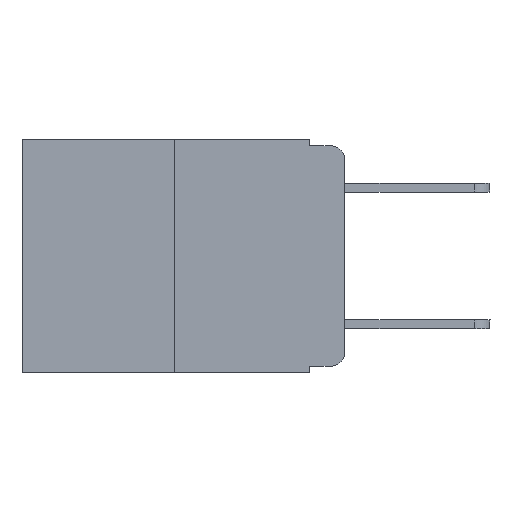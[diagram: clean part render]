
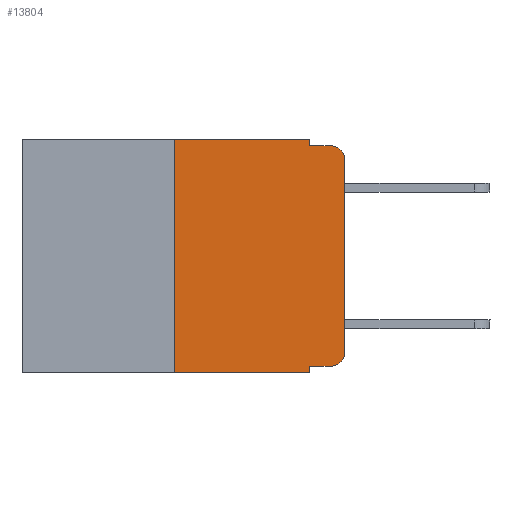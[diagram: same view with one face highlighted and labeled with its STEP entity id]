
A CAD part, left-side view. The second image highlights one B-rep face of the part: STEP entity #13804.
In plain terms, the highlighted planar face has unit normal (-1, 0, 0).
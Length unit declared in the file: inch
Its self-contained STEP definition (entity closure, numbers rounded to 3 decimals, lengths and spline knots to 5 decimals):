
#73 = LINE ( 'NONE', #9291, #13751 ) ;
#338 = CARTESIAN_POINT ( 'NONE',  ( 0., 0.051, -0.333 ) ) ;
#714 = CARTESIAN_POINT ( 'NONE',  ( 0., 0.051, -0.01 ) ) ;
#1310 = VECTOR ( 'NONE', #9167, 39.37008 ) ;
#1351 = DIRECTION ( 'NONE',  ( 0., 0., 1. ) ) ;
#1710 = DIRECTION ( 'NONE',  ( 0., 0., -1. ) ) ;
#1842 = DIRECTION ( 'NONE',  ( 0., -1., 0. ) ) ;
#2491 = VECTOR ( 'NONE', #1351, 39.37008 ) ;
#2723 = ORIENTED_EDGE ( 'NONE', *, *, #17517, .T. ) ;
#2746 = VERTEX_POINT ( 'NONE', #16112 ) ;
#2777 = LINE ( 'NONE', #2870, #3507 ) ;
#2870 = CARTESIAN_POINT ( 'NONE',  ( 0., 0., 0. ) ) ;
#2898 = LINE ( 'NONE', #4456, #6827 ) ;
#3000 = DIRECTION ( 'NONE',  ( 0., -1., 0. ) ) ;
#3030 = CARTESIAN_POINT ( 'NONE',  ( 0., 0.25, 0. ) ) ;
#3351 = CARTESIAN_POINT ( 'NONE',  ( 0., 0.473, -0.343 ) ) ;
#3507 = VECTOR ( 'NONE', #4040, 39.37008 ) ;
#3524 = ORIENTED_EDGE ( 'NONE', *, *, #6237, .F. ) ;
#3719 = CARTESIAN_POINT ( 'NONE',  ( 0., 0.051, -0.343 ) ) ;
#4040 = DIRECTION ( 'NONE',  ( 0., 0., 1. ) ) ;
#4456 = CARTESIAN_POINT ( 'NONE',  ( 0., 0.473, 0. ) ) ;
#4732 = DIRECTION ( 'NONE',  ( 0., -1., 0. ) ) ;
#4754 = CARTESIAN_POINT ( 'NONE',  ( 0., 0.02, -0.01 ) ) ;
#5245 = PLANE ( 'NONE',  #18458 ) ;
#5419 = EDGE_CURVE ( 'NONE', #12582, #6068, #6224, .T. ) ;
#5441 = VERTEX_POINT ( 'NONE', #4754 ) ;
#5540 = CARTESIAN_POINT ( 'NONE',  ( 0., 0.02, -0.333 ) ) ;
#5591 = DIRECTION ( 'NONE',  ( -1., 0., 0. ) ) ;
#5622 = ORIENTED_EDGE ( 'NONE', *, *, #15862, .T. ) ;
#5897 = CARTESIAN_POINT ( 'NONE',  ( 0., 0.25, -0.343 ) ) ;
#6068 = VERTEX_POINT ( 'NONE', #5540 ) ;
#6167 = EDGE_CURVE ( 'NONE', #13225, #5441, #10087, .T. ) ;
#6224 = LINE ( 'NONE', #338, #1310 ) ;
#6237 = EDGE_CURVE ( 'NONE', #12582, #12912, #10534, .T. ) ;
#6246 = CARTESIAN_POINT ( 'NONE',  ( 0., 0., -0.03 ) ) ;
#6281 = VERTEX_POINT ( 'NONE', #714 ) ;
#6393 = EDGE_CURVE ( 'NONE', #10237, #13225, #2777, .T. ) ;
#6550 = VERTEX_POINT ( 'NONE', #7550 ) ;
#6827 = VECTOR ( 'NONE', #3000, 39.37008 ) ;
#7256 = DIRECTION ( 'NONE',  ( 0., 0., -1. ) ) ;
#7339 = ORIENTED_EDGE ( 'NONE', *, *, #12325, .F. ) ;
#7550 = CARTESIAN_POINT ( 'NONE',  ( 0., 0.25, 0. ) ) ;
#7867 = ORIENTED_EDGE ( 'NONE', *, *, #11841, .F. ) ;
#7882 = DIRECTION ( 'NONE',  ( 1., 0., 0. ) ) ;
#7972 = CIRCLE ( 'NONE', #18930, 0.02 ) ;
#8246 = EDGE_LOOP ( 'NONE', ( #17833, #18821, #12612, #15974, #7339, #7867, #2723, #3524, #14779, #5622 ) ) ;
#8765 = EDGE_CURVE ( 'NONE', #2746, #6281, #16450, .T. ) ;
#8828 = VECTOR ( 'NONE', #16516, 39.37008 ) ;
#9167 = DIRECTION ( 'NONE',  ( 0., -1., 0. ) ) ;
#9256 = DIRECTION ( 'NONE',  ( -1., 0., 0. ) ) ;
#9291 = CARTESIAN_POINT ( 'NONE',  ( 0., 0.051, -0.01 ) ) ;
#9558 = CARTESIAN_POINT ( 'NONE',  ( 0., 0.473, 0. ) ) ;
#10087 = CIRCLE ( 'NONE', #16979, 0.02 ) ;
#10237 = VERTEX_POINT ( 'NONE', #12542 ) ;
#10465 = CARTESIAN_POINT ( 'NONE',  ( 0., 0.051, 0. ) ) ;
#10534 = LINE ( 'NONE', #11999, #8828 ) ;
#11841 = EDGE_CURVE ( 'NONE', #14480, #6550, #16453, .T. ) ;
#11999 = CARTESIAN_POINT ( 'NONE',  ( 0., 0.051, 0. ) ) ;
#12325 = EDGE_CURVE ( 'NONE', #6550, #2746, #2898, .T. ) ;
#12542 = CARTESIAN_POINT ( 'NONE',  ( 0., 0., -0.313 ) ) ;
#12582 = VERTEX_POINT ( 'NONE', #15648 ) ;
#12595 = FACE_OUTER_BOUND ( 'NONE', #8246, .T. ) ;
#12612 = ORIENTED_EDGE ( 'NONE', *, *, #13231, .F. ) ;
#12912 = VERTEX_POINT ( 'NONE', #3719 ) ;
#13225 = VERTEX_POINT ( 'NONE', #6246 ) ;
#13231 = EDGE_CURVE ( 'NONE', #6281, #5441, #73, .T. ) ;
#13751 = VECTOR ( 'NONE', #1842, 39.37008 ) ;
#13804 = ADVANCED_FACE ( 'NONE', ( #12595 ), #5245, .F. ) ;
#13948 = LINE ( 'NONE', #3351, #15455 ) ;
#14480 = VERTEX_POINT ( 'NONE', #5897 ) ;
#14779 = ORIENTED_EDGE ( 'NONE', *, *, #5419, .T. ) ;
#15070 = DIRECTION ( 'NONE',  ( 0., 0., -1. ) ) ;
#15339 = CARTESIAN_POINT ( 'NONE',  ( 0., 0.02, -0.03 ) ) ;
#15455 = VECTOR ( 'NONE', #4732, 39.37008 ) ;
#15648 = CARTESIAN_POINT ( 'NONE',  ( 0., 0.051, -0.333 ) ) ;
#15862 = EDGE_CURVE ( 'NONE', #6068, #10237, #7972, .T. ) ;
#15974 = ORIENTED_EDGE ( 'NONE', *, *, #8765, .F. ) ;
#16112 = CARTESIAN_POINT ( 'NONE',  ( 0., 0.051, 0. ) ) ;
#16450 = LINE ( 'NONE', #10465, #17921 ) ;
#16453 = LINE ( 'NONE', #3030, #2491 ) ;
#16516 = DIRECTION ( 'NONE',  ( 0., 0., -1. ) ) ;
#16979 = AXIS2_PLACEMENT_3D ( 'NONE', #15339, #9256, #1710 ) ;
#17003 = DIRECTION ( 'NONE',  ( 0., 0., -1. ) ) ;
#17355 = CARTESIAN_POINT ( 'NONE',  ( 0., 0.02, -0.313 ) ) ;
#17517 = EDGE_CURVE ( 'NONE', #14480, #12912, #13948, .T. ) ;
#17833 = ORIENTED_EDGE ( 'NONE', *, *, #6393, .T. ) ;
#17921 = VECTOR ( 'NONE', #15070, 39.37008 ) ;
#18458 = AXIS2_PLACEMENT_3D ( 'NONE', #9558, #7882, #17003 ) ;
#18821 = ORIENTED_EDGE ( 'NONE', *, *, #6167, .T. ) ;
#18930 = AXIS2_PLACEMENT_3D ( 'NONE', #17355, #5591, #7256 ) ;
